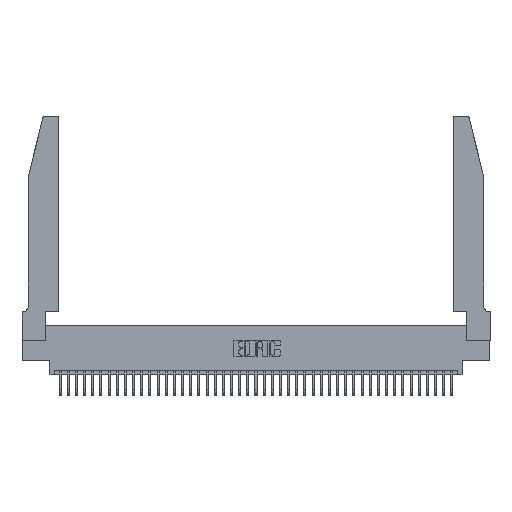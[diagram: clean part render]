
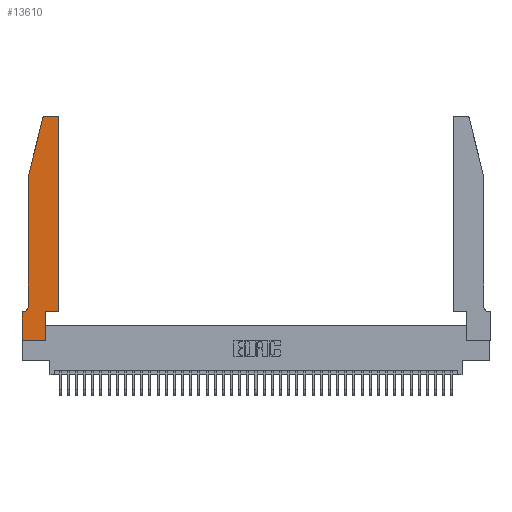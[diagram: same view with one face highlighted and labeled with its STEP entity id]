
A CAD part, top view. The second image highlights one B-rep face of the part: STEP entity #13610.
In plain terms, the highlighted planar face has unit normal (0, 0, 1).
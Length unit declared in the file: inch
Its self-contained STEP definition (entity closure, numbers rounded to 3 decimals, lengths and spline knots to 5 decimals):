
#26 = ORIENTED_EDGE ( 'NONE', *, *, #37282, .T. ) ;
#118 = VERTEX_POINT ( 'NONE', #33568 ) ;
#286 = EDGE_CURVE ( 'NONE', #7256, #23550, #40841, .T. ) ;
#613 = ORIENTED_EDGE ( 'NONE', *, *, #39380, .T. ) ;
#957 = CARTESIAN_POINT ( 'NONE',  ( 0.0755, 2., 0.37 ) ) ;
#1133 = CARTESIAN_POINT ( 'NONE',  ( 0.2605, 2.75, 0.37 ) ) ;
#1265 = VECTOR ( 'NONE', #18234, 39.37008 ) ;
#1585 = CARTESIAN_POINT ( 'NONE',  ( 0.2865, 0.35, 0.37 ) ) ;
#1856 = VECTOR ( 'NONE', #12448, 39.37008 ) ;
#2005 = VERTEX_POINT ( 'NONE', #37720 ) ;
#2402 = LINE ( 'NONE', #1133, #1265 ) ;
#2514 = EDGE_CURVE ( 'NONE', #43401, #26286, #22573, .T. ) ;
#2829 = CARTESIAN_POINT ( 'NONE',  ( 0.2865, 0.35, 0.37 ) ) ;
#3470 = CARTESIAN_POINT ( 'NONE',  ( 0.0755, 2., 0.37 ) ) ;
#3818 = EDGE_CURVE ( 'NONE', #31968, #28121, #2402, .T. ) ;
#3914 = EDGE_CURVE ( 'NONE', #41536, #43401, #26871, .T. ) ;
#6564 = CARTESIAN_POINT ( 'NONE',  ( 0.4205, 2.75, 0.37 ) ) ;
#6721 = DIRECTION ( 'NONE',  ( 1., 0., 0. ) ) ;
#7256 = VERTEX_POINT ( 'NONE', #13664 ) ;
#7612 = ORIENTED_EDGE ( 'NONE', *, *, #3818, .T. ) ;
#7737 = DIRECTION ( 'NONE',  ( 0., 0., -1. ) ) ;
#8258 = ORIENTED_EDGE ( 'NONE', *, *, #23832, .T. ) ;
#8571 = ORIENTED_EDGE ( 'NONE', *, *, #286, .T. ) ;
#9558 = EDGE_CURVE ( 'NONE', #41097, #118, #23092, .T. ) ;
#9831 = DIRECTION ( 'NONE',  ( 0., 0., 1. ) ) ;
#9958 = AXIS2_PLACEMENT_3D ( 'NONE', #24036, #7737, #19266 ) ;
#10457 = DIRECTION ( 'NONE',  ( 1., 0., 0. ) ) ;
#10707 = ORIENTED_EDGE ( 'NONE', *, *, #3914, .T. ) ;
#10852 = CARTESIAN_POINT ( 'NONE',  ( 0.284, 2.75, 0.37 ) ) ;
#10853 = CARTESIAN_POINT ( 'NONE',  ( 0.4205, 2.72, 0.37 ) ) ;
#11407 = DIRECTION ( 'NONE',  ( 1., 0., 0. ) ) ;
#12164 = EDGE_LOOP ( 'NONE', ( #7612, #8258, #18675, #26, #10707, #19923, #613, #8571, #24761, #38228, #21042, #24124 ) ) ;
#12448 = DIRECTION ( 'NONE',  ( -1., 0., 0. ) ) ;
#12476 = DIRECTION ( 'NONE',  ( 0., 1., 0. ) ) ;
#13161 = LINE ( 'NONE', #18170, #21059 ) ;
#13610 = ADVANCED_FACE ( 'NONE', ( #23803 ), #30629, .T. ) ;
#13664 = CARTESIAN_POINT ( 'NONE',  ( 0., 0., 0.37 ) ) ;
#14908 = CARTESIAN_POINT ( 'NONE',  ( 0.0755, 0.42, 0.37 ) ) ;
#15967 = LINE ( 'NONE', #40678, #33019 ) ;
#16573 = VECTOR ( 'NONE', #12476, 39.37008 ) ;
#17026 = CARTESIAN_POINT ( 'NONE',  ( 0.4505, 0.35, 0.37 ) ) ;
#18170 = CARTESIAN_POINT ( 'NONE',  ( 0.4505, 0.35, 0.37 ) ) ;
#18234 = DIRECTION ( 'NONE',  ( -1., 0., 0. ) ) ;
#18675 = ORIENTED_EDGE ( 'NONE', *, *, #9558, .T. ) ;
#19215 = CARTESIAN_POINT ( 'NONE',  ( 0.0755, 0.35, 0.37 ) ) ;
#19237 = CARTESIAN_POINT ( 'NONE',  ( 0.25487, 2.72718, 0.37 ) ) ;
#19266 = DIRECTION ( 'NONE',  ( -1., 0., 0. ) ) ;
#19923 = ORIENTED_EDGE ( 'NONE', *, *, #2514, .T. ) ;
#19932 = DIRECTION ( 'NONE',  ( 0., -1., 0. ) ) ;
#20633 = DIRECTION ( 'NONE',  ( 0., 0., 1. ) ) ;
#21042 = ORIENTED_EDGE ( 'NONE', *, *, #37978, .T. ) ;
#21059 = VECTOR ( 'NONE', #11407, 39.37008 ) ;
#21186 = DIRECTION ( 'NONE',  ( 1., 0., 0. ) ) ;
#22401 = LINE ( 'NONE', #3470, #37300 ) ;
#22573 = LINE ( 'NONE', #19215, #1856 ) ;
#22878 = AXIS2_PLACEMENT_3D ( 'NONE', #10853, #20633, #10457 ) ;
#23092 = LINE ( 'NONE', #957, #39646 ) ;
#23550 = VERTEX_POINT ( 'NONE', #32838 ) ;
#23651 = CIRCLE ( 'NONE', #22878, 0.03 ) ;
#23803 = FACE_OUTER_BOUND ( 'NONE', #12164, .T. ) ;
#23832 = EDGE_CURVE ( 'NONE', #28121, #41097, #25218, .T. ) ;
#23848 = DIRECTION ( 'NONE',  ( 1., 0., 0. ) ) ;
#24036 = CARTESIAN_POINT ( 'NONE',  ( 0.0055, 0.42, 0.37 ) ) ;
#24124 = ORIENTED_EDGE ( 'NONE', *, *, #31395, .T. ) ;
#24657 = CARTESIAN_POINT ( 'NONE',  ( 0., 0., 0.37 ) ) ;
#24761 = ORIENTED_EDGE ( 'NONE', *, *, #42651, .T. ) ;
#25218 = CIRCLE ( 'NONE', #36365, 0.03 ) ;
#25906 = LINE ( 'NONE', #26412, #32335 ) ;
#26286 = VERTEX_POINT ( 'NONE', #37813 ) ;
#26412 = CARTESIAN_POINT ( 'NONE',  ( 0., 0., 0.37 ) ) ;
#26624 = AXIS2_PLACEMENT_3D ( 'NONE', #26879, #9831, #6721 ) ;
#26871 = CIRCLE ( 'NONE', #9958, 0.07 ) ;
#26879 = CARTESIAN_POINT ( 'NONE',  ( 0., 0.35, 0.37 ) ) ;
#28121 = VERTEX_POINT ( 'NONE', #10852 ) ;
#30279 = CARTESIAN_POINT ( 'NONE',  ( 0.0055, 0.35, 0.37 ) ) ;
#30404 = EDGE_CURVE ( 'NONE', #38686, #35047, #13161, .T. ) ;
#30629 = PLANE ( 'NONE',  #26624 ) ;
#31395 = EDGE_CURVE ( 'NONE', #2005, #31968, #23651, .T. ) ;
#31968 = VERTEX_POINT ( 'NONE', #6564 ) ;
#32335 = VECTOR ( 'NONE', #33249, 39.37008 ) ;
#32838 = CARTESIAN_POINT ( 'NONE',  ( 0.2865, 0., 0.37 ) ) ;
#33019 = VECTOR ( 'NONE', #40939, 39.37008 ) ;
#33249 = DIRECTION ( 'NONE',  ( 0., -1., 0. ) ) ;
#33568 = CARTESIAN_POINT ( 'NONE',  ( 0.0755, 2., 0.37 ) ) ;
#35047 = VERTEX_POINT ( 'NONE', #17026 ) ;
#36365 = AXIS2_PLACEMENT_3D ( 'NONE', #41253, #41398, #21186 ) ;
#37282 = EDGE_CURVE ( 'NONE', #118, #41536, #22401, .T. ) ;
#37300 = VECTOR ( 'NONE', #19932, 39.37008 ) ;
#37720 = CARTESIAN_POINT ( 'NONE',  ( 0.4505, 2.72, 0.37 ) ) ;
#37813 = CARTESIAN_POINT ( 'NONE',  ( 0., 0.35, 0.37 ) ) ;
#37978 = EDGE_CURVE ( 'NONE', #35047, #2005, #15967, .T. ) ;
#38228 = ORIENTED_EDGE ( 'NONE', *, *, #30404, .T. ) ;
#38686 = VERTEX_POINT ( 'NONE', #2829 ) ;
#39380 = EDGE_CURVE ( 'NONE', #26286, #7256, #25906, .T. ) ;
#39646 = VECTOR ( 'NONE', #41866, 39.37008 ) ;
#40678 = CARTESIAN_POINT ( 'NONE',  ( 0.4505, 0.35, 0.37 ) ) ;
#40841 = LINE ( 'NONE', #24657, #43041 ) ;
#40939 = DIRECTION ( 'NONE',  ( 0., 1., 0. ) ) ;
#41097 = VERTEX_POINT ( 'NONE', #19237 ) ;
#41253 = CARTESIAN_POINT ( 'NONE',  ( 0.284, 2.72, 0.37 ) ) ;
#41398 = DIRECTION ( 'NONE',  ( 0., 0., 1. ) ) ;
#41536 = VERTEX_POINT ( 'NONE', #14908 ) ;
#41866 = DIRECTION ( 'NONE',  ( -0.239, -0.971, 0. ) ) ;
#42064 = LINE ( 'NONE', #1585, #16573 ) ;
#42651 = EDGE_CURVE ( 'NONE', #23550, #38686, #42064, .T. ) ;
#43041 = VECTOR ( 'NONE', #23848, 39.37008 ) ;
#43401 = VERTEX_POINT ( 'NONE', #30279 ) ;
